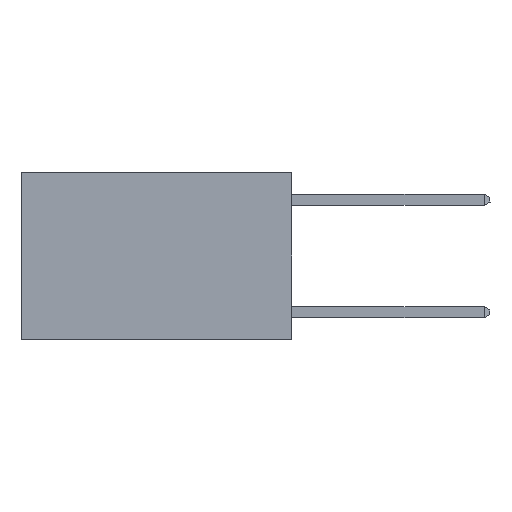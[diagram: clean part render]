
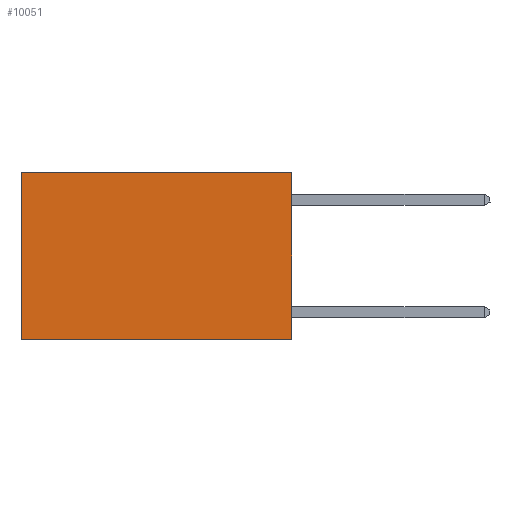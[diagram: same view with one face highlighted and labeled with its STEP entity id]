
A CAD part, left-side view. The second image highlights one B-rep face of the part: STEP entity #10051.
In plain terms, the highlighted planar face has unit normal (-1, 0, 0).
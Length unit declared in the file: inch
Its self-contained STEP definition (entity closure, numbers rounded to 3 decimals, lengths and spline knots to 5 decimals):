
#1514 = CARTESIAN_POINT ( 'NONE',  ( 0.2625, 0., 0. ) ) ;
#2029 = VECTOR ( 'NONE', #21429, 39.37008 ) ;
#3276 = CARTESIAN_POINT ( 'NONE',  ( 0.2625, 0., 0. ) ) ;
#4803 = AXIS2_PLACEMENT_3D ( 'NONE', #1514, #10718, #11460 ) ;
#5746 = CARTESIAN_POINT ( 'NONE',  ( 0.2625, 0.6, -0.37 ) ) ;
#6134 = VERTEX_POINT ( 'NONE', #7099 ) ;
#6963 = EDGE_CURVE ( 'NONE', #26780, #27473, #10984, .T. ) ;
#7099 = CARTESIAN_POINT ( 'NONE',  ( 0.2625, 0., -0.37 ) ) ;
#7776 = VECTOR ( 'NONE', #24763, 39.37008 ) ;
#7814 = CARTESIAN_POINT ( 'NONE',  ( 0.2625, 0., -0.37 ) ) ;
#8805 = CARTESIAN_POINT ( 'NONE',  ( 0.2625, 0., 0. ) ) ;
#8954 = LINE ( 'NONE', #8805, #21297 ) ;
#10051 = ADVANCED_FACE ( 'NONE', ( #19766 ), #22189, .F. ) ;
#10718 = DIRECTION ( 'NONE',  ( 1., 0., 0. ) ) ;
#10984 = LINE ( 'NONE', #19887, #16784 ) ;
#11460 = DIRECTION ( 'NONE',  ( 0., 0., -1. ) ) ;
#13338 = DIRECTION ( 'NONE',  ( 0., 1., 0. ) ) ;
#15338 = ORIENTED_EDGE ( 'NONE', *, *, #28972, .F. ) ;
#15707 = LINE ( 'NONE', #20092, #7776 ) ;
#16784 = VECTOR ( 'NONE', #22440, 39.37008 ) ;
#18615 = CARTESIAN_POINT ( 'NONE',  ( 0.2625, 0.6, 0. ) ) ;
#18666 = VERTEX_POINT ( 'NONE', #3276 ) ;
#19766 = FACE_OUTER_BOUND ( 'NONE', #29721, .T. ) ;
#19887 = CARTESIAN_POINT ( 'NONE',  ( 0.2625, 0.6, 0. ) ) ;
#20092 = CARTESIAN_POINT ( 'NONE',  ( 0.2625, 0., 0. ) ) ;
#21297 = VECTOR ( 'NONE', #13338, 39.37008 ) ;
#21429 = DIRECTION ( 'NONE',  ( 0., 1., 0. ) ) ;
#22189 = PLANE ( 'NONE',  #4803 ) ;
#22440 = DIRECTION ( 'NONE',  ( 0., 0., -1. ) ) ;
#23193 = ORIENTED_EDGE ( 'NONE', *, *, #28715, .F. ) ;
#23544 = LINE ( 'NONE', #7814, #2029 ) ;
#24763 = DIRECTION ( 'NONE',  ( 0., 0., -1. ) ) ;
#25495 = ORIENTED_EDGE ( 'NONE', *, *, #6963, .T. ) ;
#26004 = ORIENTED_EDGE ( 'NONE', *, *, #28168, .T. ) ;
#26780 = VERTEX_POINT ( 'NONE', #18615 ) ;
#27473 = VERTEX_POINT ( 'NONE', #5746 ) ;
#28168 = EDGE_CURVE ( 'NONE', #18666, #26780, #8954, .T. ) ;
#28715 = EDGE_CURVE ( 'NONE', #18666, #6134, #15707, .T. ) ;
#28972 = EDGE_CURVE ( 'NONE', #6134, #27473, #23544, .T. ) ;
#29721 = EDGE_LOOP ( 'NONE', ( #25495, #15338, #23193, #26004 ) ) ;
